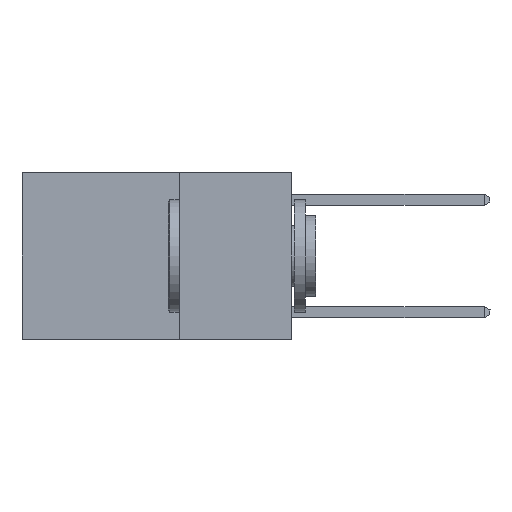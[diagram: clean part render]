
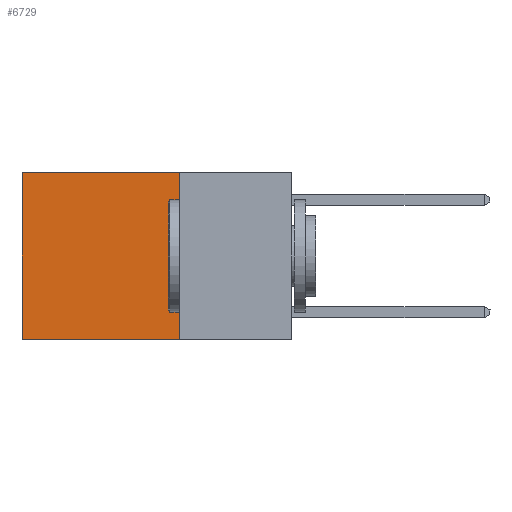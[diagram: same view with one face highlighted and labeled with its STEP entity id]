
A CAD part, left-side view. The second image highlights one B-rep face of the part: STEP entity #6729.
In plain terms, the highlighted planar face has unit normal (-1, 0, 0).
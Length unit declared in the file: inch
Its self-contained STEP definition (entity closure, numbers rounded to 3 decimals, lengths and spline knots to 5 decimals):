
#30 = FACE_OUTER_BOUND ( 'NONE', #3219, .T. ) ;
#47 = VECTOR ( 'NONE', #591, 39.37008 ) ;
#380 = LINE ( 'NONE', #9001, #47 ) ;
#591 = DIRECTION ( 'NONE',  ( 0., 1., 0. ) ) ;
#966 = ORIENTED_EDGE ( 'NONE', *, *, #4351, .T. ) ;
#999 = ORIENTED_EDGE ( 'NONE', *, *, #2487, .F. ) ;
#1043 = ORIENTED_EDGE ( 'NONE', *, *, #6721, .F. ) ;
#1160 = ORIENTED_EDGE ( 'NONE', *, *, #10401, .T. ) ;
#1864 = VERTEX_POINT ( 'NONE', #5601 ) ;
#2275 = AXIS2_PLACEMENT_3D ( 'NONE', #3212, #8308, #3243 ) ;
#2487 = EDGE_CURVE ( 'NONE', #1864, #3911, #8438, .T. ) ;
#3212 = CARTESIAN_POINT ( 'NONE',  ( 0.2625, 0.25, 0. ) ) ;
#3219 = EDGE_LOOP ( 'NONE', ( #966, #999, #1043, #1160 ) ) ;
#3243 = DIRECTION ( 'NONE',  ( 0., 0., -1. ) ) ;
#3911 = VERTEX_POINT ( 'NONE', #10501 ) ;
#4073 = DIRECTION ( 'NONE',  ( 0., 0., -1. ) ) ;
#4342 = LINE ( 'NONE', #6212, #10346 ) ;
#4351 = EDGE_CURVE ( 'NONE', #5950, #3911, #4342, .T. ) ;
#4682 = VECTOR ( 'NONE', #4073, 39.37008 ) ;
#5601 = CARTESIAN_POINT ( 'NONE',  ( 0.2625, 0.25, -0.37 ) ) ;
#5950 = VERTEX_POINT ( 'NONE', #6483 ) ;
#6212 = CARTESIAN_POINT ( 'NONE',  ( 0.2625, 0.6, 0. ) ) ;
#6417 = DIRECTION ( 'NONE',  ( 0., 1., 0. ) ) ;
#6483 = CARTESIAN_POINT ( 'NONE',  ( 0.2625, 0.6, 0. ) ) ;
#6721 = EDGE_CURVE ( 'NONE', #7502, #1864, #6890, .T. ) ;
#6729 = ADVANCED_FACE ( 'NONE', ( #30 ), #10618, .F. ) ;
#6890 = LINE ( 'NONE', #10582, #4682 ) ;
#7502 = VERTEX_POINT ( 'NONE', #9952 ) ;
#8308 = DIRECTION ( 'NONE',  ( 1., 0., 0. ) ) ;
#8438 = LINE ( 'NONE', #9677, #10248 ) ;
#9001 = CARTESIAN_POINT ( 'NONE',  ( 0.2625, 0.25, 0. ) ) ;
#9677 = CARTESIAN_POINT ( 'NONE',  ( 0.2625, 0.25, -0.37 ) ) ;
#9952 = CARTESIAN_POINT ( 'NONE',  ( 0.2625, 0.25, 0. ) ) ;
#10248 = VECTOR ( 'NONE', #6417, 39.37008 ) ;
#10257 = DIRECTION ( 'NONE',  ( 0., 0., -1. ) ) ;
#10346 = VECTOR ( 'NONE', #10257, 39.37008 ) ;
#10401 = EDGE_CURVE ( 'NONE', #7502, #5950, #380, .T. ) ;
#10501 = CARTESIAN_POINT ( 'NONE',  ( 0.2625, 0.6, -0.37 ) ) ;
#10582 = CARTESIAN_POINT ( 'NONE',  ( 0.2625, 0.25, 0. ) ) ;
#10618 = PLANE ( 'NONE',  #2275 ) ;
